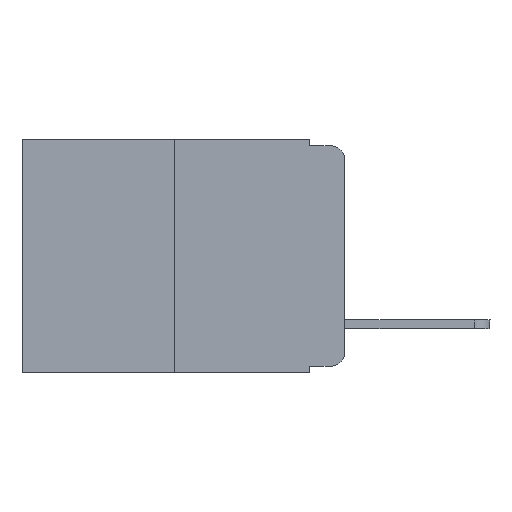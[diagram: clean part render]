
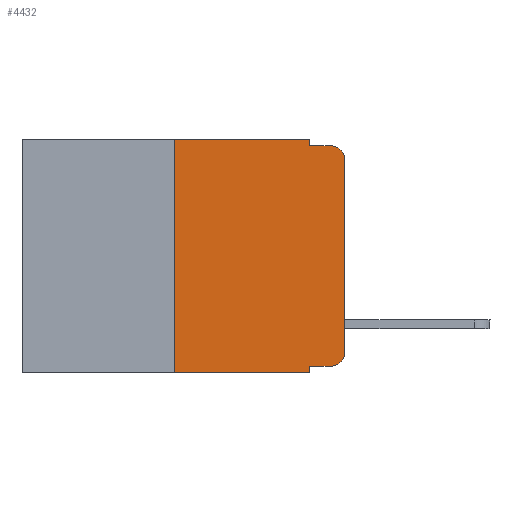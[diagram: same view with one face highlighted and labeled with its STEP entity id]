
A CAD part, left-side view. The second image highlights one B-rep face of the part: STEP entity #4432.
In plain terms, the highlighted planar face has unit normal (-1, 0, 0).
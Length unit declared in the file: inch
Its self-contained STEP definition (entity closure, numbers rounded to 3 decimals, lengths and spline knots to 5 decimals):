
#262 = CARTESIAN_POINT ( 'NONE',  ( 0., 0.25, 0. ) ) ;
#303 = CIRCLE ( 'NONE', #11065, 0.02 ) ;
#522 = CARTESIAN_POINT ( 'NONE',  ( 0., 0.051, 0. ) ) ;
#1024 = LINE ( 'NONE', #12229, #7194 ) ;
#1157 = CARTESIAN_POINT ( 'NONE',  ( 0., 0.473, -0.343 ) ) ;
#1454 = ORIENTED_EDGE ( 'NONE', *, *, #20827, .F. ) ;
#1659 = CIRCLE ( 'NONE', #21177, 0.02 ) ;
#2508 = LINE ( 'NONE', #10112, #3302 ) ;
#2571 = EDGE_LOOP ( 'NONE', ( #11145, #14279, #21287, #1454, #21663, #15066, #4266, #12401, #14034, #15238 ) ) ;
#2766 = DIRECTION ( 'NONE',  ( 0., 0., 1. ) ) ;
#3302 = VECTOR ( 'NONE', #17722, 39.37008 ) ;
#4266 = ORIENTED_EDGE ( 'NONE', *, *, #19134, .T. ) ;
#4293 = VECTOR ( 'NONE', #7560, 39.37008 ) ;
#4432 = ADVANCED_FACE ( 'NONE', ( #22533 ), #7185, .F. ) ;
#4621 = LINE ( 'NONE', #19475, #7687 ) ;
#5609 = CARTESIAN_POINT ( 'NONE',  ( 0., 0.25, -0.343 ) ) ;
#5651 = EDGE_CURVE ( 'NONE', #21557, #16662, #23584, .T. ) ;
#6440 = CARTESIAN_POINT ( 'NONE',  ( 0., 0.02, -0.333 ) ) ;
#6864 = VERTEX_POINT ( 'NONE', #6440 ) ;
#7185 = PLANE ( 'NONE',  #23674 ) ;
#7194 = VECTOR ( 'NONE', #2766, 39.37008 ) ;
#7560 = DIRECTION ( 'NONE',  ( 0., -1., 0. ) ) ;
#7687 = VECTOR ( 'NONE', #12214, 39.37008 ) ;
#7957 = VERTEX_POINT ( 'NONE', #11320 ) ;
#7980 = CARTESIAN_POINT ( 'NONE',  ( 0., 0.051, 0. ) ) ;
#7987 = VERTEX_POINT ( 'NONE', #17292 ) ;
#8267 = VECTOR ( 'NONE', #16329, 39.37008 ) ;
#8601 = CARTESIAN_POINT ( 'NONE',  ( 0., 0.02, -0.313 ) ) ;
#8924 = VECTOR ( 'NONE', #21477, 39.37008 ) ;
#9041 = DIRECTION ( 'NONE',  ( 1., 0., 0. ) ) ;
#9991 = LINE ( 'NONE', #522, #8924 ) ;
#10112 = CARTESIAN_POINT ( 'NONE',  ( 0., 0.25, 0. ) ) ;
#10438 = VERTEX_POINT ( 'NONE', #5609 ) ;
#10717 = CARTESIAN_POINT ( 'NONE',  ( 0., 0.051, -0.01 ) ) ;
#11042 = CARTESIAN_POINT ( 'NONE',  ( 0., 0.473, 0. ) ) ;
#11065 = AXIS2_PLACEMENT_3D ( 'NONE', #8601, #14696, #23831 ) ;
#11145 = ORIENTED_EDGE ( 'NONE', *, *, #12861, .T. ) ;
#11320 = CARTESIAN_POINT ( 'NONE',  ( 0., 0., -0.03 ) ) ;
#11847 = VERTEX_POINT ( 'NONE', #262 ) ;
#12214 = DIRECTION ( 'NONE',  ( 0., -1., 0. ) ) ;
#12229 = CARTESIAN_POINT ( 'NONE',  ( 0., 0., 0. ) ) ;
#12401 = ORIENTED_EDGE ( 'NONE', *, *, #5651, .F. ) ;
#12861 = EDGE_CURVE ( 'NONE', #14312, #7957, #1024, .T. ) ;
#13285 = LINE ( 'NONE', #15292, #4293 ) ;
#13321 = VECTOR ( 'NONE', #15587, 39.37008 ) ;
#13355 = EDGE_CURVE ( 'NONE', #7957, #20779, #1659, .T. ) ;
#14034 = ORIENTED_EDGE ( 'NONE', *, *, #15470, .T. ) ;
#14279 = ORIENTED_EDGE ( 'NONE', *, *, #13355, .T. ) ;
#14312 = VERTEX_POINT ( 'NONE', #22473 ) ;
#14572 = CARTESIAN_POINT ( 'NONE',  ( 0., 0.02, -0.03 ) ) ;
#14657 = DIRECTION ( 'NONE',  ( 0., 0., -1. ) ) ;
#14696 = DIRECTION ( 'NONE',  ( -1., 0., 0. ) ) ;
#14991 = EDGE_CURVE ( 'NONE', #7987, #20779, #20321, .T. ) ;
#15010 = EDGE_CURVE ( 'NONE', #6864, #14312, #303, .T. ) ;
#15066 = ORIENTED_EDGE ( 'NONE', *, *, #19516, .F. ) ;
#15238 = ORIENTED_EDGE ( 'NONE', *, *, #15010, .T. ) ;
#15292 = CARTESIAN_POINT ( 'NONE',  ( 0., 0.051, -0.333 ) ) ;
#15470 = EDGE_CURVE ( 'NONE', #21557, #6864, #13285, .T. ) ;
#15484 = CARTESIAN_POINT ( 'NONE',  ( 0., 0.051, 0. ) ) ;
#15587 = DIRECTION ( 'NONE',  ( 0., 0., -1. ) ) ;
#16043 = VECTOR ( 'NONE', #24106, 39.37008 ) ;
#16329 = DIRECTION ( 'NONE',  ( 0., -1., 0. ) ) ;
#16662 = VERTEX_POINT ( 'NONE', #20295 ) ;
#17292 = CARTESIAN_POINT ( 'NONE',  ( 0., 0.051, -0.01 ) ) ;
#17722 = DIRECTION ( 'NONE',  ( 0., 0., 1. ) ) ;
#17842 = CARTESIAN_POINT ( 'NONE',  ( 0., 0.02, -0.01 ) ) ;
#19134 = EDGE_CURVE ( 'NONE', #10438, #16662, #24343, .T. ) ;
#19446 = EDGE_CURVE ( 'NONE', #11847, #23749, #4621, .T. ) ;
#19475 = CARTESIAN_POINT ( 'NONE',  ( 0., 0.473, 0. ) ) ;
#19516 = EDGE_CURVE ( 'NONE', #10438, #11847, #2508, .T. ) ;
#20295 = CARTESIAN_POINT ( 'NONE',  ( 0., 0.051, -0.343 ) ) ;
#20321 = LINE ( 'NONE', #10717, #8267 ) ;
#20779 = VERTEX_POINT ( 'NONE', #17842 ) ;
#20827 = EDGE_CURVE ( 'NONE', #23749, #7987, #9991, .T. ) ;
#21043 = CARTESIAN_POINT ( 'NONE',  ( 0., 0.051, -0.333 ) ) ;
#21177 = AXIS2_PLACEMENT_3D ( 'NONE', #14572, #23949, #22314 ) ;
#21287 = ORIENTED_EDGE ( 'NONE', *, *, #14991, .F. ) ;
#21477 = DIRECTION ( 'NONE',  ( 0., 0., -1. ) ) ;
#21557 = VERTEX_POINT ( 'NONE', #21043 ) ;
#21663 = ORIENTED_EDGE ( 'NONE', *, *, #19446, .F. ) ;
#22314 = DIRECTION ( 'NONE',  ( 0., 0., -1. ) ) ;
#22473 = CARTESIAN_POINT ( 'NONE',  ( 0., 0., -0.313 ) ) ;
#22533 = FACE_OUTER_BOUND ( 'NONE', #2571, .T. ) ;
#23584 = LINE ( 'NONE', #7980, #13321 ) ;
#23674 = AXIS2_PLACEMENT_3D ( 'NONE', #11042, #9041, #14657 ) ;
#23749 = VERTEX_POINT ( 'NONE', #15484 ) ;
#23831 = DIRECTION ( 'NONE',  ( 0., 0., -1. ) ) ;
#23949 = DIRECTION ( 'NONE',  ( -1., 0., 0. ) ) ;
#24106 = DIRECTION ( 'NONE',  ( 0., -1., 0. ) ) ;
#24343 = LINE ( 'NONE', #1157, #16043 ) ;
